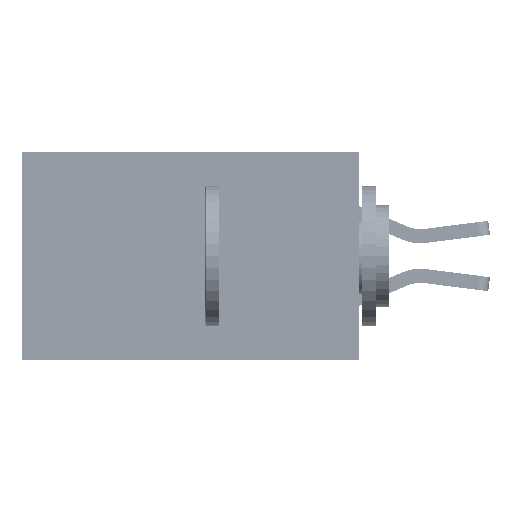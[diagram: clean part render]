
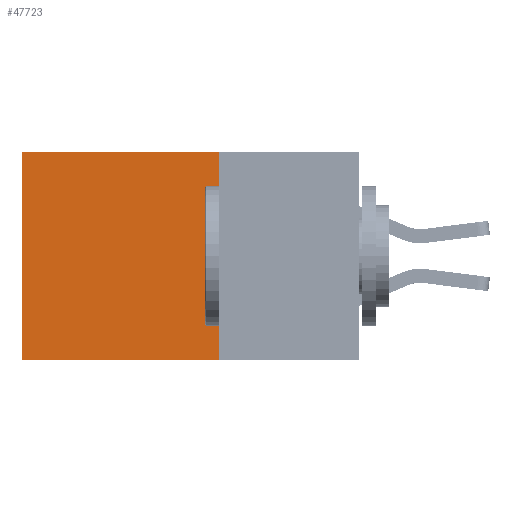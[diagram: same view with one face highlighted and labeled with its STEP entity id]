
A CAD part, left-side view. The second image highlights one B-rep face of the part: STEP entity #47723.
In plain terms, the highlighted planar face has unit normal (-1, 0, 0).
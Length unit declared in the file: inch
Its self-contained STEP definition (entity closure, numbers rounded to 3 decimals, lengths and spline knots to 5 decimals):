
#711 = AXIS2_PLACEMENT_3D ( 'NONE', #14944, #33377, #44719 ) ;
#993 = VERTEX_POINT ( 'NONE', #43732 ) ;
#1376 = CARTESIAN_POINT ( 'NONE',  ( 0.2875, 0.6, 0. ) ) ;
#1802 = VERTEX_POINT ( 'NONE', #41858 ) ;
#6994 = VERTEX_POINT ( 'NONE', #29555 ) ;
#8560 = VECTOR ( 'NONE', #28029, 39.37008 ) ;
#9687 = EDGE_CURVE ( 'NONE', #6994, #46262, #16378, .T. ) ;
#9873 = ORIENTED_EDGE ( 'NONE', *, *, #11340, .F. ) ;
#11340 = EDGE_CURVE ( 'NONE', #993, #1802, #36039, .T. ) ;
#13024 = CARTESIAN_POINT ( 'NONE',  ( 0.2875, 0.6, 0. ) ) ;
#13897 = VECTOR ( 'NONE', #47283, 39.37008 ) ;
#14912 = EDGE_LOOP ( 'NONE', ( #23919, #9873, #18623, #18531 ) ) ;
#14944 = CARTESIAN_POINT ( 'NONE',  ( 0.2875, 0.25, 0. ) ) ;
#16378 = LINE ( 'NONE', #21461, #42023 ) ;
#18531 = ORIENTED_EDGE ( 'NONE', *, *, #9687, .T. ) ;
#18623 = ORIENTED_EDGE ( 'NONE', *, *, #44848, .F. ) ;
#18948 = VECTOR ( 'NONE', #36630, 39.37008 ) ;
#21408 = CARTESIAN_POINT ( 'NONE',  ( 0.2875, 0.25, -0.37 ) ) ;
#21461 = CARTESIAN_POINT ( 'NONE',  ( 0.2875, 0.25, 0. ) ) ;
#23919 = ORIENTED_EDGE ( 'NONE', *, *, #44498, .T. ) ;
#28029 = DIRECTION ( 'NONE',  ( 0., 0., -1. ) ) ;
#29555 = CARTESIAN_POINT ( 'NONE',  ( 0.2875, 0.25, 0. ) ) ;
#32439 = FACE_OUTER_BOUND ( 'NONE', #14912, .T. ) ;
#32909 = CARTESIAN_POINT ( 'NONE',  ( 0.2875, 0.25, 0. ) ) ;
#33377 = DIRECTION ( 'NONE',  ( 1., 0., 0. ) ) ;
#36039 = LINE ( 'NONE', #21408, #13897 ) ;
#36630 = DIRECTION ( 'NONE',  ( 0., 0., -1. ) ) ;
#36965 = PLANE ( 'NONE',  #711 ) ;
#38158 = LINE ( 'NONE', #32909, #18948 ) ;
#41858 = CARTESIAN_POINT ( 'NONE',  ( 0.2875, 0.6, -0.37 ) ) ;
#42023 = VECTOR ( 'NONE', #47499, 39.37008 ) ;
#43732 = CARTESIAN_POINT ( 'NONE',  ( 0.2875, 0.25, -0.37 ) ) ;
#44498 = EDGE_CURVE ( 'NONE', #46262, #1802, #47587, .T. ) ;
#44719 = DIRECTION ( 'NONE',  ( 0., 0., -1. ) ) ;
#44848 = EDGE_CURVE ( 'NONE', #6994, #993, #38158, .T. ) ;
#46262 = VERTEX_POINT ( 'NONE', #1376 ) ;
#47283 = DIRECTION ( 'NONE',  ( 0., 1., 0. ) ) ;
#47499 = DIRECTION ( 'NONE',  ( 0., 1., 0. ) ) ;
#47587 = LINE ( 'NONE', #13024, #8560 ) ;
#47723 = ADVANCED_FACE ( 'NONE', ( #32439 ), #36965, .F. ) ;
